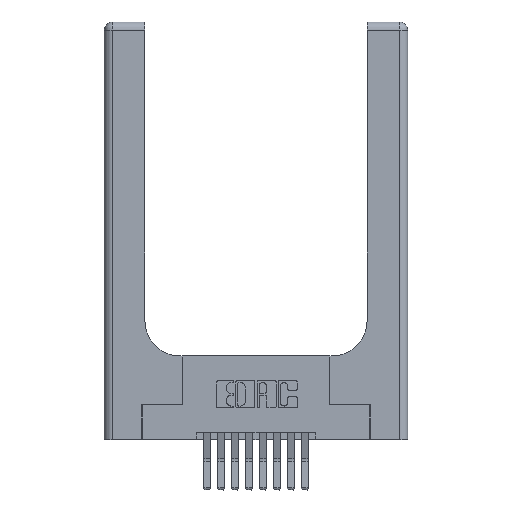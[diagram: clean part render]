
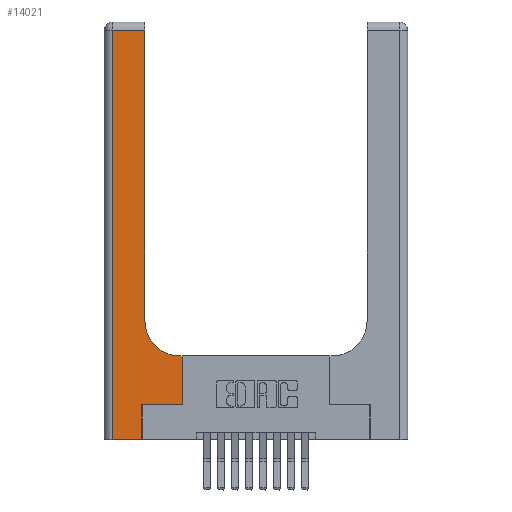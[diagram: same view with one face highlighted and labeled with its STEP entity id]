
A CAD part, top view. The second image highlights one B-rep face of the part: STEP entity #14021.
In plain terms, the highlighted planar face has unit normal (0, 0, 1).
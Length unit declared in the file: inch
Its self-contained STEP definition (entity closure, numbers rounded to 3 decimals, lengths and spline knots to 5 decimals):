
#330 = CARTESIAN_POINT ( 'NONE',  ( 0.269, 0., 0.37 ) ) ;
#722 = VERTEX_POINT ( 'NONE', #13489 ) ;
#973 = DIRECTION ( 'NONE',  ( 0., 1., 0. ) ) ;
#1111 = CARTESIAN_POINT ( 'NONE',  ( 0., 3., 0.37 ) ) ;
#1151 = EDGE_CURVE ( 'NONE', #9082, #4824, #11045, .T. ) ;
#1264 = ORIENTED_EDGE ( 'NONE', *, *, #6896, .T. ) ;
#1318 = DIRECTION ( 'NONE',  ( 1., 0., 0. ) ) ;
#1489 = CARTESIAN_POINT ( 'NONE',  ( 0.269, 0.25, 0.37 ) ) ;
#1724 = ORIENTED_EDGE ( 'NONE', *, *, #10391, .T. ) ;
#1861 = VERTEX_POINT ( 'NONE', #10835 ) ;
#1970 = CARTESIAN_POINT ( 'NONE',  ( 0.269, 0., 0.37 ) ) ;
#1971 = LINE ( 'NONE', #13074, #15412 ) ;
#2024 = CARTESIAN_POINT ( 'NONE',  ( 0.06, 3., 0.37 ) ) ;
#2299 = ORIENTED_EDGE ( 'NONE', *, *, #16146, .T. ) ;
#2324 = LINE ( 'NONE', #13044, #11897 ) ;
#2333 = ORIENTED_EDGE ( 'NONE', *, *, #13562, .T. ) ;
#2662 = DIRECTION ( 'NONE',  ( 1., 0., 0. ) ) ;
#2781 = FACE_OUTER_BOUND ( 'NONE', #14722, .T. ) ;
#3073 = LINE ( 'NONE', #5065, #8343 ) ;
#3087 = DIRECTION ( 'NONE',  ( -1., 0., 0. ) ) ;
#3321 = VERTEX_POINT ( 'NONE', #7597 ) ;
#3406 = LINE ( 'NONE', #14235, #9058 ) ;
#3498 = DIRECTION ( 'NONE',  ( 1., 0., 0. ) ) ;
#3538 = VECTOR ( 'NONE', #1318, 39.37008 ) ;
#3838 = CARTESIAN_POINT ( 'NONE',  ( 0.5585, 0.6, 0.37 ) ) ;
#4036 = ORIENTED_EDGE ( 'NONE', *, *, #11206, .T. ) ;
#4736 = AXIS2_PLACEMENT_3D ( 'NONE', #1111, #16153, #6100 ) ;
#4824 = VERTEX_POINT ( 'NONE', #7050 ) ;
#5065 = CARTESIAN_POINT ( 'NONE',  ( 0.269, 0.25, 0.37 ) ) ;
#6100 = DIRECTION ( 'NONE',  ( -1., 0., 0. ) ) ;
#6659 = LINE ( 'NONE', #1970, #8206 ) ;
#6773 = ORIENTED_EDGE ( 'NONE', *, *, #1151, .T. ) ;
#6896 = EDGE_CURVE ( 'NONE', #15381, #9082, #2324, .T. ) ;
#7050 = CARTESIAN_POINT ( 'NONE',  ( 0.06, 0., 0.37 ) ) ;
#7247 = CARTESIAN_POINT ( 'NONE',  ( 0.2915, 0.6, 0.37 ) ) ;
#7249 = AXIS2_PLACEMENT_3D ( 'NONE', #11075, #14825, #3498 ) ;
#7461 = CARTESIAN_POINT ( 'NONE',  ( 0.2915, 2.94, 0.37 ) ) ;
#7597 = CARTESIAN_POINT ( 'NONE',  ( 0.2915, 0.85, 0.37 ) ) ;
#8206 = VECTOR ( 'NONE', #13119, 39.37008 ) ;
#8287 = DIRECTION ( 'NONE',  ( 0., -1., 0. ) ) ;
#8343 = VECTOR ( 'NONE', #2662, 39.37008 ) ;
#9058 = VECTOR ( 'NONE', #9186, 39.37008 ) ;
#9082 = VERTEX_POINT ( 'NONE', #14116 ) ;
#9186 = DIRECTION ( 'NONE',  ( 0., 1., 0. ) ) ;
#10152 = VERTEX_POINT ( 'NONE', #3838 ) ;
#10300 = VERTEX_POINT ( 'NONE', #1489 ) ;
#10391 = EDGE_CURVE ( 'NONE', #10152, #722, #11784, .T. ) ;
#10835 = CARTESIAN_POINT ( 'NONE',  ( 0.5585, 0.25, 0.37 ) ) ;
#10893 = ORIENTED_EDGE ( 'NONE', *, *, #15573, .T. ) ;
#11002 = CIRCLE ( 'NONE', #7249, 0.25 ) ;
#11045 = LINE ( 'NONE', #2024, #14555 ) ;
#11075 = CARTESIAN_POINT ( 'NONE',  ( 0.5415, 0.85, 0.37 ) ) ;
#11206 = EDGE_CURVE ( 'NONE', #10300, #1861, #3073, .T. ) ;
#11383 = CARTESIAN_POINT ( 'NONE',  ( 0., 0., 0.37 ) ) ;
#11784 = LINE ( 'NONE', #7247, #14144 ) ;
#11897 = VECTOR ( 'NONE', #3087, 39.37008 ) ;
#12858 = EDGE_CURVE ( 'NONE', #3321, #15381, #3406, .T. ) ;
#13044 = CARTESIAN_POINT ( 'NONE',  ( 0., 2.94, 0.37 ) ) ;
#13074 = CARTESIAN_POINT ( 'NONE',  ( 0.5585, 0.25, 0.37 ) ) ;
#13119 = DIRECTION ( 'NONE',  ( 0., 1., 0. ) ) ;
#13410 = DIRECTION ( 'NONE',  ( -1., 0., 0. ) ) ;
#13489 = CARTESIAN_POINT ( 'NONE',  ( 0.5415, 0.6, 0.37 ) ) ;
#13562 = EDGE_CURVE ( 'NONE', #722, #3321, #11002, .T. ) ;
#13899 = LINE ( 'NONE', #11383, #3538 ) ;
#14021 = ADVANCED_FACE ( 'NONE', ( #2781 ), #14906, .F. ) ;
#14116 = CARTESIAN_POINT ( 'NONE',  ( 0.06, 2.94, 0.37 ) ) ;
#14144 = VECTOR ( 'NONE', #13410, 39.37008 ) ;
#14235 = CARTESIAN_POINT ( 'NONE',  ( 0.2915, 3., 0.37 ) ) ;
#14290 = ORIENTED_EDGE ( 'NONE', *, *, #12858, .T. ) ;
#14555 = VECTOR ( 'NONE', #8287, 39.37008 ) ;
#14722 = EDGE_LOOP ( 'NONE', ( #14290, #1264, #6773, #10893, #14764, #4036, #2299, #1724, #2333 ) ) ;
#14751 = VERTEX_POINT ( 'NONE', #330 ) ;
#14764 = ORIENTED_EDGE ( 'NONE', *, *, #15171, .T. ) ;
#14825 = DIRECTION ( 'NONE',  ( 0., 0., -1. ) ) ;
#14906 = PLANE ( 'NONE',  #4736 ) ;
#15171 = EDGE_CURVE ( 'NONE', #14751, #10300, #6659, .T. ) ;
#15381 = VERTEX_POINT ( 'NONE', #7461 ) ;
#15412 = VECTOR ( 'NONE', #973, 39.37008 ) ;
#15573 = EDGE_CURVE ( 'NONE', #4824, #14751, #13899, .T. ) ;
#16146 = EDGE_CURVE ( 'NONE', #1861, #10152, #1971, .T. ) ;
#16153 = DIRECTION ( 'NONE',  ( 0., 0., -1. ) ) ;
